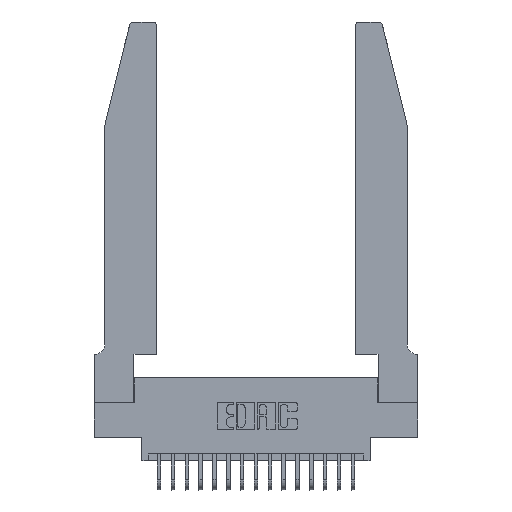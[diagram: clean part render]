
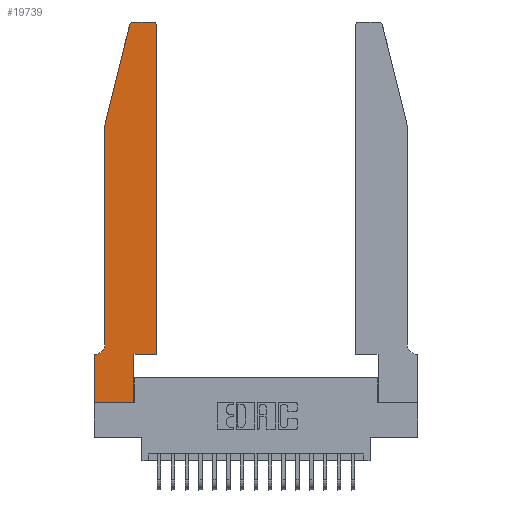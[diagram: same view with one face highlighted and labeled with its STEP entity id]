
A CAD part, top view. The second image highlights one B-rep face of the part: STEP entity #19739.
In plain terms, the highlighted planar face has unit normal (0, 0, 1).
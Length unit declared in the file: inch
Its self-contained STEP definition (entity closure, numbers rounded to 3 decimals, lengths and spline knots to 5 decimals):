
#29 = DIRECTION ( 'NONE',  ( 1., 0., 0. ) ) ;
#233 = EDGE_CURVE ( 'NONE', #4515, #19400, #6293, .T. ) ;
#248 = LINE ( 'NONE', #14439, #17854 ) ;
#500 = EDGE_CURVE ( 'NONE', #16276, #3737, #18849, .T. ) ;
#690 = EDGE_LOOP ( 'NONE', ( #4973, #9974, #1381, #14938, #1926, #15465, #2484, #11561, #12088, #12318, #21197, #17280 ) ) ;
#871 = VERTEX_POINT ( 'NONE', #2530 ) ;
#1124 = AXIS2_PLACEMENT_3D ( 'NONE', #5615, #13413, #2976 ) ;
#1308 = CARTESIAN_POINT ( 'NONE',  ( 0.2865, 0.35, 0.37 ) ) ;
#1381 = ORIENTED_EDGE ( 'NONE', *, *, #19150, .T. ) ;
#1407 = EDGE_CURVE ( 'NONE', #4752, #16276, #7582, .T. ) ;
#1582 = CARTESIAN_POINT ( 'NONE',  ( 0.0755, 2., 0.37 ) ) ;
#1635 = CARTESIAN_POINT ( 'NONE',  ( 0.4505, 0.35, 0.37 ) ) ;
#1680 = AXIS2_PLACEMENT_3D ( 'NONE', #20385, #10380, #29 ) ;
#1926 = ORIENTED_EDGE ( 'NONE', *, *, #233, .T. ) ;
#2177 = CARTESIAN_POINT ( 'NONE',  ( 0.0055, 0.35, 0.37 ) ) ;
#2215 = VECTOR ( 'NONE', #21804, 39.37008 ) ;
#2484 = ORIENTED_EDGE ( 'NONE', *, *, #10310, .T. ) ;
#2530 = CARTESIAN_POINT ( 'NONE',  ( 0.4205, 2.75, 0.37 ) ) ;
#2976 = DIRECTION ( 'NONE',  ( -1., 0., 0. ) ) ;
#3737 = VERTEX_POINT ( 'NONE', #13846 ) ;
#3832 = VECTOR ( 'NONE', #8387, 39.37008 ) ;
#3959 = CARTESIAN_POINT ( 'NONE',  ( 0., 0.35, 0.37 ) ) ;
#4065 = DIRECTION ( 'NONE',  ( 0., -1., 0. ) ) ;
#4376 = DIRECTION ( 'NONE',  ( 1., 0., 0. ) ) ;
#4515 = VERTEX_POINT ( 'NONE', #19560 ) ;
#4695 = LINE ( 'NONE', #8022, #13645 ) ;
#4704 = FACE_OUTER_BOUND ( 'NONE', #690, .T. ) ;
#4752 = VERTEX_POINT ( 'NONE', #21806 ) ;
#4973 = ORIENTED_EDGE ( 'NONE', *, *, #13938, .T. ) ;
#5048 = VECTOR ( 'NONE', #5264, 39.37008 ) ;
#5187 = CARTESIAN_POINT ( 'NONE',  ( 0.0755, 0.35, 0.37 ) ) ;
#5264 = DIRECTION ( 'NONE',  ( -1., 0., 0. ) ) ;
#5562 = CIRCLE ( 'NONE', #1680, 0.03 ) ;
#5594 = VERTEX_POINT ( 'NONE', #12170 ) ;
#5615 = CARTESIAN_POINT ( 'NONE',  ( 0.0055, 0.42, 0.37 ) ) ;
#5649 = CIRCLE ( 'NONE', #11147, 0.03 ) ;
#5663 = VERTEX_POINT ( 'NONE', #3959 ) ;
#5905 = DIRECTION ( 'NONE',  ( 0., 0., 1. ) ) ;
#6109 = DIRECTION ( 'NONE',  ( 1., 0., 0. ) ) ;
#6293 = CIRCLE ( 'NONE', #1124, 0.07 ) ;
#6531 = CARTESIAN_POINT ( 'NONE',  ( 0.4505, 0.35, 0.37 ) ) ;
#6772 = CARTESIAN_POINT ( 'NONE',  ( 0.0755, 2., 0.37 ) ) ;
#7008 = VERTEX_POINT ( 'NONE', #17226 ) ;
#7009 = CARTESIAN_POINT ( 'NONE',  ( 0., 0.35, 0.37 ) ) ;
#7081 = DIRECTION ( 'NONE',  ( 1., 0., 0. ) ) ;
#7316 = CARTESIAN_POINT ( 'NONE',  ( 0.2865, 0.35, 0.37 ) ) ;
#7374 = EDGE_CURVE ( 'NONE', #7008, #4515, #20141, .T. ) ;
#7441 = EDGE_CURVE ( 'NONE', #3737, #18885, #10724, .T. ) ;
#7582 = LINE ( 'NONE', #7316, #12003 ) ;
#8022 = CARTESIAN_POINT ( 'NONE',  ( 0.2605, 2.75, 0.37 ) ) ;
#8387 = DIRECTION ( 'NONE',  ( 0., -1., 0. ) ) ;
#9191 = DIRECTION ( 'NONE',  ( 0., 1., 0. ) ) ;
#9974 = ORIENTED_EDGE ( 'NONE', *, *, #16648, .T. ) ;
#10051 = LINE ( 'NONE', #5187, #5048 ) ;
#10310 = EDGE_CURVE ( 'NONE', #5663, #12433, #18459, .T. ) ;
#10380 = DIRECTION ( 'NONE',  ( 0., 0., 1. ) ) ;
#10724 = LINE ( 'NONE', #1635, #19117 ) ;
#10775 = EDGE_CURVE ( 'NONE', #19400, #5663, #10051, .T. ) ;
#11033 = CARTESIAN_POINT ( 'NONE',  ( 0.284, 2.75, 0.37 ) ) ;
#11147 = AXIS2_PLACEMENT_3D ( 'NONE', #15923, #5905, #17627 ) ;
#11561 = ORIENTED_EDGE ( 'NONE', *, *, #19520, .T. ) ;
#12003 = VECTOR ( 'NONE', #9191, 39.37008 ) ;
#12032 = PLANE ( 'NONE',  #21904 ) ;
#12088 = ORIENTED_EDGE ( 'NONE', *, *, #1407, .T. ) ;
#12170 = CARTESIAN_POINT ( 'NONE',  ( 0.25487, 2.72718, 0.37 ) ) ;
#12318 = ORIENTED_EDGE ( 'NONE', *, *, #500, .T. ) ;
#12433 = VERTEX_POINT ( 'NONE', #15277 ) ;
#13413 = DIRECTION ( 'NONE',  ( 0., 0., -1. ) ) ;
#13645 = VECTOR ( 'NONE', #19731, 39.37008 ) ;
#13846 = CARTESIAN_POINT ( 'NONE',  ( 0.4505, 0.35, 0.37 ) ) ;
#13938 = EDGE_CURVE ( 'NONE', #871, #17548, #4695, .T. ) ;
#14386 = VECTOR ( 'NONE', #6109, 39.37008 ) ;
#14439 = CARTESIAN_POINT ( 'NONE',  ( 0., 0., 0.37 ) ) ;
#14938 = ORIENTED_EDGE ( 'NONE', *, *, #7374, .T. ) ;
#15277 = CARTESIAN_POINT ( 'NONE',  ( 0., 0., 0.37 ) ) ;
#15465 = ORIENTED_EDGE ( 'NONE', *, *, #10775, .T. ) ;
#15740 = LINE ( 'NONE', #1582, #2215 ) ;
#15823 = CARTESIAN_POINT ( 'NONE',  ( 0., 0., 0.37 ) ) ;
#15923 = CARTESIAN_POINT ( 'NONE',  ( 0.284, 2.72, 0.37 ) ) ;
#16276 = VERTEX_POINT ( 'NONE', #1308 ) ;
#16648 = EDGE_CURVE ( 'NONE', #17548, #5594, #5649, .T. ) ;
#17065 = DIRECTION ( 'NONE',  ( 0., 0., 1. ) ) ;
#17226 = CARTESIAN_POINT ( 'NONE',  ( 0.0755, 2., 0.37 ) ) ;
#17280 = ORIENTED_EDGE ( 'NONE', *, *, #18499, .T. ) ;
#17405 = VECTOR ( 'NONE', #4065, 39.37008 ) ;
#17548 = VERTEX_POINT ( 'NONE', #11033 ) ;
#17627 = DIRECTION ( 'NONE',  ( 1., 0., 0. ) ) ;
#17854 = VECTOR ( 'NONE', #4376, 39.37008 ) ;
#18459 = LINE ( 'NONE', #15823, #17405 ) ;
#18499 = EDGE_CURVE ( 'NONE', #18885, #871, #5562, .T. ) ;
#18849 = LINE ( 'NONE', #6531, #14386 ) ;
#18885 = VERTEX_POINT ( 'NONE', #21333 ) ;
#19117 = VECTOR ( 'NONE', #21917, 39.37008 ) ;
#19150 = EDGE_CURVE ( 'NONE', #5594, #7008, #15740, .T. ) ;
#19400 = VERTEX_POINT ( 'NONE', #2177 ) ;
#19520 = EDGE_CURVE ( 'NONE', #12433, #4752, #248, .T. ) ;
#19560 = CARTESIAN_POINT ( 'NONE',  ( 0.0755, 0.42, 0.37 ) ) ;
#19731 = DIRECTION ( 'NONE',  ( -1., 0., 0. ) ) ;
#19739 = ADVANCED_FACE ( 'NONE', ( #4704 ), #12032, .T. ) ;
#20141 = LINE ( 'NONE', #6772, #3832 ) ;
#20385 = CARTESIAN_POINT ( 'NONE',  ( 0.4205, 2.72, 0.37 ) ) ;
#21197 = ORIENTED_EDGE ( 'NONE', *, *, #7441, .T. ) ;
#21333 = CARTESIAN_POINT ( 'NONE',  ( 0.4505, 2.72, 0.37 ) ) ;
#21804 = DIRECTION ( 'NONE',  ( -0.239, -0.971, 0. ) ) ;
#21806 = CARTESIAN_POINT ( 'NONE',  ( 0.2865, 0., 0.37 ) ) ;
#21904 = AXIS2_PLACEMENT_3D ( 'NONE', #7009, #17065, #7081 ) ;
#21917 = DIRECTION ( 'NONE',  ( 0., 1., 0. ) ) ;
